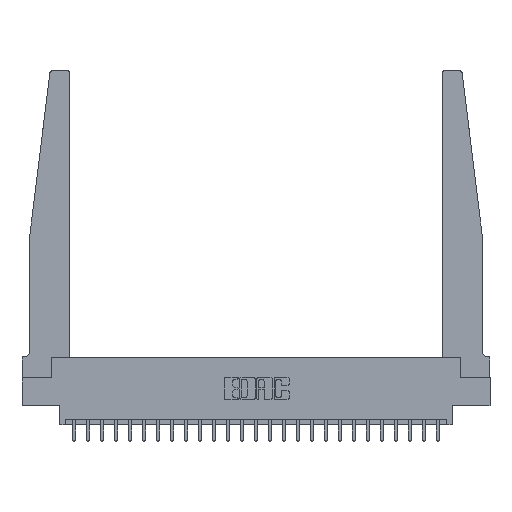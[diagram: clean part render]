
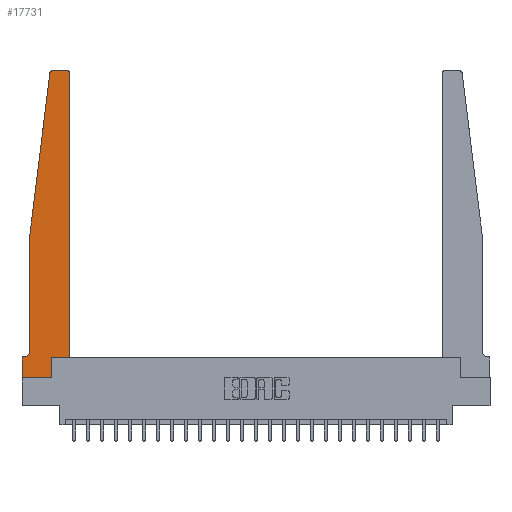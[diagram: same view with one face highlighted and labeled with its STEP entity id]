
A CAD part, top view. The second image highlights one B-rep face of the part: STEP entity #17731.
In plain terms, the highlighted planar face has unit normal (0, 0, 1).
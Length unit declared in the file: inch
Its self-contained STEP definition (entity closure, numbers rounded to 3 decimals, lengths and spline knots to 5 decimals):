
#56 = VERTEX_POINT ( 'NONE', #2365 ) ;
#249 = DIRECTION ( 'NONE',  ( 1., 0., 0. ) ) ;
#335 = EDGE_CURVE ( 'NONE', #23847, #21648, #24156, .T. ) ;
#344 = ORIENTED_EDGE ( 'NONE', *, *, #13305, .T. ) ;
#625 = ORIENTED_EDGE ( 'NONE', *, *, #10610, .T. ) ;
#779 = EDGE_CURVE ( 'NONE', #10442, #56, #15313, .T. ) ;
#818 = DIRECTION ( 'NONE',  ( 0., 1., 0. ) ) ;
#917 = CARTESIAN_POINT ( 'NONE',  ( 0., 0.1875, 0.37 ) ) ;
#1807 = PLANE ( 'NONE',  #18899 ) ;
#1967 = DIRECTION ( 'NONE',  ( -0.122, -0.992, 0. ) ) ;
#2190 = CARTESIAN_POINT ( 'NONE',  ( 0., 0., 0.37 ) ) ;
#2357 = EDGE_CURVE ( 'NONE', #3383, #13642, #23506, .T. ) ;
#2365 = CARTESIAN_POINT ( 'NONE',  ( 0.2605, 0.18, 0.37 ) ) ;
#2555 = LINE ( 'NONE', #15165, #7390 ) ;
#2557 = VECTOR ( 'NONE', #18812, 39.37008 ) ;
#2658 = DIRECTION ( 'NONE',  ( 0., 0., -1. ) ) ;
#3383 = VERTEX_POINT ( 'NONE', #6430 ) ;
#3736 = DIRECTION ( 'NONE',  ( 0., 0., 1. ) ) ;
#4591 = VECTOR ( 'NONE', #23556, 39.37008 ) ;
#5034 = CARTESIAN_POINT ( 'NONE',  ( 0.065, 0.2375, 0.37 ) ) ;
#5406 = CARTESIAN_POINT ( 'NONE',  ( 0.065, 1.25, 0.37 ) ) ;
#5424 = CARTESIAN_POINT ( 'NONE',  ( 0.2605, 0., 0.37 ) ) ;
#6430 = CARTESIAN_POINT ( 'NONE',  ( 0.425, 2.72, 0.37 ) ) ;
#6432 = VERTEX_POINT ( 'NONE', #917 ) ;
#7058 = CARTESIAN_POINT ( 'NONE',  ( 0., 0., 0.37 ) ) ;
#7390 = VECTOR ( 'NONE', #17098, 39.37008 ) ;
#7459 = VECTOR ( 'NONE', #9751, 39.37008 ) ;
#7517 = CARTESIAN_POINT ( 'NONE',  ( 0.27653, 2.72, 0.37 ) ) ;
#8395 = LINE ( 'NONE', #8697, #12884 ) ;
#8467 = EDGE_CURVE ( 'NONE', #13642, #19020, #2555, .T. ) ;
#8697 = CARTESIAN_POINT ( 'NONE',  ( 0.425, 0.18, 0.37 ) ) ;
#9315 = VECTOR ( 'NONE', #17466, 39.37008 ) ;
#9416 = DIRECTION ( 'NONE',  ( 1., 0., 0. ) ) ;
#9751 = DIRECTION ( 'NONE',  ( 0., -1., 0. ) ) ;
#10137 = EDGE_CURVE ( 'NONE', #21648, #20717, #10770, .T. ) ;
#10213 = CARTESIAN_POINT ( 'NONE',  ( 0.015, 0.1875, 0.37 ) ) ;
#10288 = VECTOR ( 'NONE', #818, 39.37008 ) ;
#10337 = FACE_OUTER_BOUND ( 'NONE', #19501, .T. ) ;
#10442 = VERTEX_POINT ( 'NONE', #5424 ) ;
#10610 = EDGE_CURVE ( 'NONE', #6432, #22860, #12533, .T. ) ;
#10635 = DIRECTION ( 'NONE',  ( 1., 0., 0. ) ) ;
#10770 = CIRCLE ( 'NONE', #22571, 0.05 ) ;
#11028 = CARTESIAN_POINT ( 'NONE',  ( 0.27653, 2.75, 0.37 ) ) ;
#11273 = CARTESIAN_POINT ( 'NONE',  ( 0.425, 0.18, 0.37 ) ) ;
#11725 = DIRECTION ( 'NONE',  ( 0., 0., 1. ) ) ;
#12533 = LINE ( 'NONE', #19225, #7459 ) ;
#12884 = VECTOR ( 'NONE', #10635, 39.37008 ) ;
#12898 = AXIS2_PLACEMENT_3D ( 'NONE', #7517, #20803, #9416 ) ;
#13305 = EDGE_CURVE ( 'NONE', #22409, #3383, #22789, .T. ) ;
#13642 = VERTEX_POINT ( 'NONE', #14308 ) ;
#14099 = CARTESIAN_POINT ( 'NONE',  ( 0.015, 0.2375, 0.37 ) ) ;
#14112 = CARTESIAN_POINT ( 'NONE',  ( 0.2605, 0.18, 0.37 ) ) ;
#14308 = CARTESIAN_POINT ( 'NONE',  ( 0.395, 2.75, 0.37 ) ) ;
#14465 = VECTOR ( 'NONE', #19635, 39.37008 ) ;
#14839 = VERTEX_POINT ( 'NONE', #21809 ) ;
#14899 = CARTESIAN_POINT ( 'NONE',  ( 0.425, 0.18, 0.37 ) ) ;
#15048 = LINE ( 'NONE', #21536, #14465 ) ;
#15165 = CARTESIAN_POINT ( 'NONE',  ( 0.25, 2.75, 0.37 ) ) ;
#15209 = CIRCLE ( 'NONE', #12898, 0.03 ) ;
#15313 = LINE ( 'NONE', #14112, #10288 ) ;
#15966 = EDGE_CURVE ( 'NONE', #14839, #23847, #21200, .T. ) ;
#15983 = DIRECTION ( 'NONE',  ( -1., 0., 0. ) ) ;
#16136 = VECTOR ( 'NONE', #1967, 39.37008 ) ;
#17085 = DIRECTION ( 'NONE',  ( 1., 0., 0. ) ) ;
#17098 = DIRECTION ( 'NONE',  ( -1., 0., 0. ) ) ;
#17272 = AXIS2_PLACEMENT_3D ( 'NONE', #23034, #11725, #249 ) ;
#17466 = DIRECTION ( 'NONE',  ( 1., 0., 0. ) ) ;
#17731 = ADVANCED_FACE ( 'NONE', ( #10337 ), #1807, .T. ) ;
#18028 = EDGE_CURVE ( 'NONE', #20717, #6432, #15048, .T. ) ;
#18728 = ORIENTED_EDGE ( 'NONE', *, *, #21106, .T. ) ;
#18812 = DIRECTION ( 'NONE',  ( 0., 1., 0. ) ) ;
#18899 = AXIS2_PLACEMENT_3D ( 'NONE', #20719, #3736, #17085 ) ;
#19020 = VERTEX_POINT ( 'NONE', #11028 ) ;
#19148 = CARTESIAN_POINT ( 'NONE',  ( 0.065, 1.25, 0.37 ) ) ;
#19225 = CARTESIAN_POINT ( 'NONE',  ( 0., 0., 0.37 ) ) ;
#19501 = EDGE_LOOP ( 'NONE', ( #19813, #18728, #19975, #20726, #20798, #21157, #625, #21472, #22941, #22687, #344, #24404 ) ) ;
#19635 = DIRECTION ( 'NONE',  ( -1., 0., 0. ) ) ;
#19813 = ORIENTED_EDGE ( 'NONE', *, *, #8467, .T. ) ;
#19975 = ORIENTED_EDGE ( 'NONE', *, *, #15966, .T. ) ;
#19984 = EDGE_CURVE ( 'NONE', #22860, #10442, #20025, .T. ) ;
#20025 = LINE ( 'NONE', #2190, #9315 ) ;
#20278 = EDGE_CURVE ( 'NONE', #56, #22409, #8395, .T. ) ;
#20717 = VERTEX_POINT ( 'NONE', #10213 ) ;
#20719 = CARTESIAN_POINT ( 'NONE',  ( 0., 0.1875, 0.37 ) ) ;
#20726 = ORIENTED_EDGE ( 'NONE', *, *, #335, .T. ) ;
#20798 = ORIENTED_EDGE ( 'NONE', *, *, #10137, .T. ) ;
#20803 = DIRECTION ( 'NONE',  ( 0., 0., 1. ) ) ;
#21106 = EDGE_CURVE ( 'NONE', #19020, #14839, #15209, .T. ) ;
#21157 = ORIENTED_EDGE ( 'NONE', *, *, #18028, .T. ) ;
#21200 = LINE ( 'NONE', #19148, #16136 ) ;
#21472 = ORIENTED_EDGE ( 'NONE', *, *, #19984, .T. ) ;
#21536 = CARTESIAN_POINT ( 'NONE',  ( 0.065, 0.1875, 0.37 ) ) ;
#21648 = VERTEX_POINT ( 'NONE', #5034 ) ;
#21809 = CARTESIAN_POINT ( 'NONE',  ( 0.24675, 2.72367, 0.37 ) ) ;
#22409 = VERTEX_POINT ( 'NONE', #14899 ) ;
#22571 = AXIS2_PLACEMENT_3D ( 'NONE', #14099, #2658, #15983 ) ;
#22687 = ORIENTED_EDGE ( 'NONE', *, *, #20278, .T. ) ;
#22789 = LINE ( 'NONE', #11273, #2557 ) ;
#22860 = VERTEX_POINT ( 'NONE', #7058 ) ;
#22941 = ORIENTED_EDGE ( 'NONE', *, *, #779, .T. ) ;
#23034 = CARTESIAN_POINT ( 'NONE',  ( 0.395, 2.72, 0.37 ) ) ;
#23300 = CARTESIAN_POINT ( 'NONE',  ( 0.065, 1.25, 0.37 ) ) ;
#23506 = CIRCLE ( 'NONE', #17272, 0.03 ) ;
#23556 = DIRECTION ( 'NONE',  ( 0., -1., 0. ) ) ;
#23847 = VERTEX_POINT ( 'NONE', #23300 ) ;
#24156 = LINE ( 'NONE', #5406, #4591 ) ;
#24404 = ORIENTED_EDGE ( 'NONE', *, *, #2357, .T. ) ;
